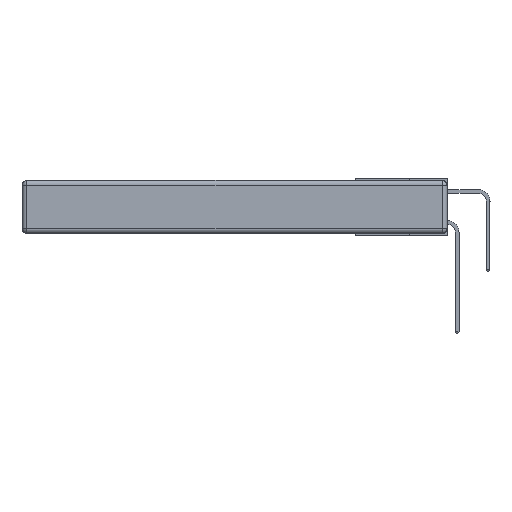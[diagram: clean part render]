
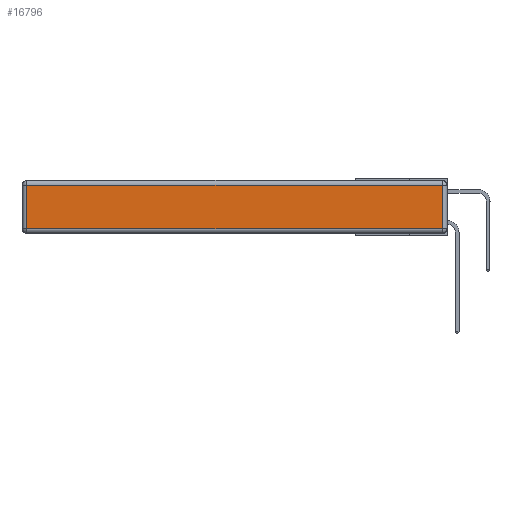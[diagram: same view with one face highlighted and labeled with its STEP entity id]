
A CAD part, left-side view. The second image highlights one B-rep face of the part: STEP entity #16796.
In plain terms, the highlighted planar face has unit normal (-1, 0, 0).
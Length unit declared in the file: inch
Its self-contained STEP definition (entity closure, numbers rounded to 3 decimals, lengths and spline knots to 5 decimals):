
#356 = VERTEX_POINT ( 'NONE', #27370 ) ;
#1030 = VECTOR ( 'NONE', #20612, 39.37008 ) ;
#1488 = ORIENTED_EDGE ( 'NONE', *, *, #31216, .T. ) ;
#2957 = EDGE_CURVE ( 'NONE', #5582, #13014, #7416, .T. ) ;
#4081 = VECTOR ( 'NONE', #13659, 39.37008 ) ;
#4966 = CARTESIAN_POINT ( 'NONE',  ( 0., 0., -0.343 ) ) ;
#5582 = VERTEX_POINT ( 'NONE', #25422 ) ;
#7073 = LINE ( 'NONE', #15282, #25923 ) ;
#7416 = LINE ( 'NONE', #9675, #25467 ) ;
#8928 = FACE_OUTER_BOUND ( 'NONE', #17917, .T. ) ;
#9209 = CARTESIAN_POINT ( 'NONE',  ( 0., 0.03, -0.03 ) ) ;
#9675 = CARTESIAN_POINT ( 'NONE',  ( 0., 0.03, -0.343 ) ) ;
#9905 = CARTESIAN_POINT ( 'NONE',  ( 0., 2.72, -0.313 ) ) ;
#12703 = LINE ( 'NONE', #12779, #1030 ) ;
#12779 = CARTESIAN_POINT ( 'NONE',  ( 0., 0., -0.313 ) ) ;
#13014 = VERTEX_POINT ( 'NONE', #9209 ) ;
#13551 = CARTESIAN_POINT ( 'NONE',  ( 0., 2.75, -0.03 ) ) ;
#13659 = DIRECTION ( 'NONE',  ( 0., 1., 0. ) ) ;
#14850 = DIRECTION ( 'NONE',  ( 0., 0., 1. ) ) ;
#15282 = CARTESIAN_POINT ( 'NONE',  ( 0., 2.72, -0.343 ) ) ;
#16796 = ADVANCED_FACE ( 'NONE', ( #8928 ), #27740, .T. ) ;
#17883 = EDGE_CURVE ( 'NONE', #23911, #5582, #12703, .T. ) ;
#17917 = EDGE_LOOP ( 'NONE', ( #31707, #32576, #25757, #1488 ) ) ;
#20612 = DIRECTION ( 'NONE',  ( 0., -1., 0. ) ) ;
#23256 = AXIS2_PLACEMENT_3D ( 'NONE', #4966, #25156, #30314 ) ;
#23911 = VERTEX_POINT ( 'NONE', #9905 ) ;
#25156 = DIRECTION ( 'NONE',  ( -1., 0., 0. ) ) ;
#25422 = CARTESIAN_POINT ( 'NONE',  ( 0., 0.03, -0.313 ) ) ;
#25467 = VECTOR ( 'NONE', #14850, 39.37008 ) ;
#25757 = ORIENTED_EDGE ( 'NONE', *, *, #26055, .T. ) ;
#25923 = VECTOR ( 'NONE', #28117, 39.37008 ) ;
#26055 = EDGE_CURVE ( 'NONE', #13014, #356, #26983, .T. ) ;
#26983 = LINE ( 'NONE', #13551, #4081 ) ;
#27370 = CARTESIAN_POINT ( 'NONE',  ( 0., 2.72, -0.03 ) ) ;
#27740 = PLANE ( 'NONE',  #23256 ) ;
#28117 = DIRECTION ( 'NONE',  ( 0., 0., -1. ) ) ;
#30314 = DIRECTION ( 'NONE',  ( 0., 0., 1. ) ) ;
#31216 = EDGE_CURVE ( 'NONE', #356, #23911, #7073, .T. ) ;
#31707 = ORIENTED_EDGE ( 'NONE', *, *, #17883, .T. ) ;
#32576 = ORIENTED_EDGE ( 'NONE', *, *, #2957, .T. ) ;
